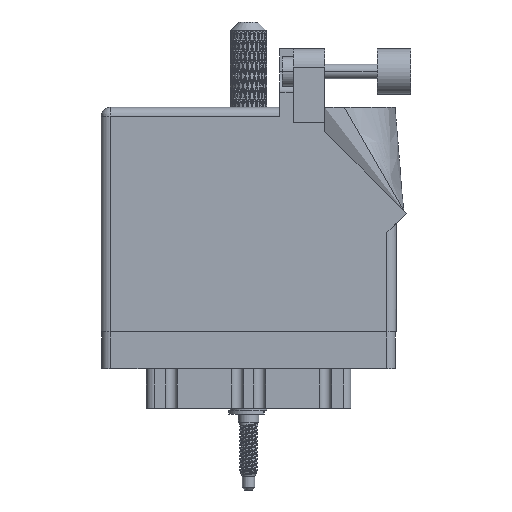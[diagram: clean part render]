
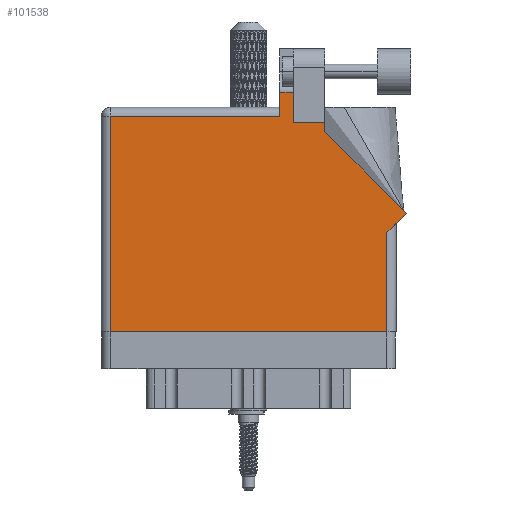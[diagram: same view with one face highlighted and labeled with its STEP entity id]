
A CAD part, front view. The second image highlights one B-rep face of the part: STEP entity #101538.
In plain terms, the highlighted face is planar.
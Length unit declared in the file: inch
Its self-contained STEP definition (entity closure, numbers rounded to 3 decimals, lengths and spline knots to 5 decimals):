
#59 = DIRECTION ( 'NONE',  ( -1., 0., 0. ) ) ;
#2060 = VERTEX_POINT ( 'NONE', #86287 ) ;
#2966 = CARTESIAN_POINT ( 'NONE',  ( 1.948, 0.675, 0. ) ) ;
#5149 = CARTESIAN_POINT ( 'NONE',  ( 2.08071, 0.80771, 0. ) ) ;
#6017 = EDGE_CURVE ( 'NONE', #79848, #96081, #8811, .T. ) ;
#7831 = ORIENTED_EDGE ( 'NONE', *, *, #81977, .T. ) ;
#8289 = CARTESIAN_POINT ( 'NONE',  ( 0., 1.468, 0. ) ) ;
#8692 = CARTESIAN_POINT ( 'NONE',  ( 0.062, 1.468, 0. ) ) ;
#8811 = LINE ( 'NONE', #8289, #60024 ) ;
#11763 = EDGE_CURVE ( 'NONE', #2060, #68552, #32461, .T. ) ;
#12787 = VECTOR ( 'NONE', #89440, 39.37008 ) ;
#12826 = VERTEX_POINT ( 'NONE', #76459 ) ;
#13745 = VECTOR ( 'NONE', #19058, 39.37008 ) ;
#13921 = LINE ( 'NONE', #80703, #87282 ) ;
#13922 = CARTESIAN_POINT ( 'NONE',  ( 0., 1.53, 0. ) ) ;
#14000 = ORIENTED_EDGE ( 'NONE', *, *, #46606, .T. ) ;
#14435 = PLANE ( 'NONE',  #76879 ) ;
#14499 = VECTOR ( 'NONE', #88847, 39.37008 ) ;
#15387 = ORIENTED_EDGE ( 'NONE', *, *, #80254, .T. ) ;
#15699 = LINE ( 'NONE', #31146, #12787 ) ;
#18017 = CARTESIAN_POINT ( 'NONE',  ( 1.524, 1.36442, 0. ) ) ;
#19058 = DIRECTION ( 'NONE',  ( 0., 1., 0. ) ) ;
#19302 = CARTESIAN_POINT ( 'NONE',  ( 1.311, 1.43, 0. ) ) ;
#19380 = LINE ( 'NONE', #28450, #73697 ) ;
#22245 = CARTESIAN_POINT ( 'NONE',  ( 2.08071, 0.80771, 0. ) ) ;
#24450 = EDGE_CURVE ( 'NONE', #85967, #58935, #13921, .T. ) ;
#26199 = ORIENTED_EDGE ( 'NONE', *, *, #64897, .T. ) ;
#26257 = LINE ( 'NONE', #19302, #26749 ) ;
#26749 = VECTOR ( 'NONE', #43212, 39.37008 ) ;
#28450 = CARTESIAN_POINT ( 'NONE',  ( 1.948, 0.737, 0. ) ) ;
#29911 = EDGE_CURVE ( 'NONE', #47731, #33781, #68970, .T. ) ;
#31067 = EDGE_CURVE ( 'NONE', #58935, #2060, #26257, .T. ) ;
#31146 = CARTESIAN_POINT ( 'NONE',  ( 0.062, 0., 0. ) ) ;
#31417 = FACE_OUTER_BOUND ( 'NONE', #61093, .T. ) ;
#32461 = LINE ( 'NONE', #50458, #50585 ) ;
#33781 = VERTEX_POINT ( 'NONE', #96773 ) ;
#35774 = ORIENTED_EDGE ( 'NONE', *, *, #31067, .T. ) ;
#37519 = DIRECTION ( 'NONE',  ( -0.707, 0.707, 0. ) ) ;
#40652 = DIRECTION ( 'NONE',  ( -1., 0., 0. ) ) ;
#43212 = DIRECTION ( 'NONE',  ( 0., 1., 0. ) ) ;
#43459 = ORIENTED_EDGE ( 'NONE', *, *, #24450, .T. ) ;
#45478 = LINE ( 'NONE', #5149, #87457 ) ;
#46606 = EDGE_CURVE ( 'NONE', #12826, #85967, #59933, .T. ) ;
#47731 = VERTEX_POINT ( 'NONE', #70955 ) ;
#50458 = CARTESIAN_POINT ( 'NONE',  ( 1.64177, 1.6315, 0. ) ) ;
#50585 = VECTOR ( 'NONE', #59, 39.37008 ) ;
#50645 = LINE ( 'NONE', #82974, #14499 ) ;
#52094 = VECTOR ( 'NONE', #56704, 39.37008 ) ;
#52248 = EDGE_CURVE ( 'NONE', #102484, #54928, #50645, .T. ) ;
#54928 = VERTEX_POINT ( 'NONE', #22245 ) ;
#56704 = DIRECTION ( 'NONE',  ( 0., -1., 0. ) ) ;
#58935 = VERTEX_POINT ( 'NONE', #88009 ) ;
#59933 = LINE ( 'NONE', #18017, #13745 ) ;
#60024 = VECTOR ( 'NONE', #40652, 39.37008 ) ;
#61093 = EDGE_LOOP ( 'NONE', ( #35774, #104684, #83140, #97493, #15387, #91819, #26199, #81775, #7831, #14000, #43459 ) ) ;
#61824 = DIRECTION ( 'NONE',  ( 0., 1., 0. ) ) ;
#64897 = EDGE_CURVE ( 'NONE', #33781, #102484, #19380, .T. ) ;
#65742 = LINE ( 'NONE', #97522, #52094 ) ;
#68552 = VERTEX_POINT ( 'NONE', #92241 ) ;
#68970 = LINE ( 'NONE', #86425, #104150 ) ;
#70955 = CARTESIAN_POINT ( 'NONE',  ( 0.062, 0., 0. ) ) ;
#73697 = VECTOR ( 'NONE', #61824, 39.37008 ) ;
#76459 = CARTESIAN_POINT ( 'NONE',  ( 1.524, 1.36442, 0. ) ) ;
#76879 = AXIS2_PLACEMENT_3D ( 'NONE', #13922, #94527, #96593 ) ;
#79848 = VERTEX_POINT ( 'NONE', #92431 ) ;
#80254 = EDGE_CURVE ( 'NONE', #96081, #47731, #15699, .T. ) ;
#80703 = CARTESIAN_POINT ( 'NONE',  ( 1.524, 1.43, 0. ) ) ;
#81775 = ORIENTED_EDGE ( 'NONE', *, *, #52248, .T. ) ;
#81977 = EDGE_CURVE ( 'NONE', #54928, #12826, #45478, .T. ) ;
#82974 = CARTESIAN_POINT ( 'NONE',  ( 2.01, 0.737, 0. ) ) ;
#83140 = ORIENTED_EDGE ( 'NONE', *, *, #89285, .T. ) ;
#85967 = VERTEX_POINT ( 'NONE', #93219 ) ;
#86287 = CARTESIAN_POINT ( 'NONE',  ( 1.311, 1.6315, 0. ) ) ;
#86425 = CARTESIAN_POINT ( 'NONE',  ( 0., 0., 0. ) ) ;
#87282 = VECTOR ( 'NONE', #95558, 39.37008 ) ;
#87457 = VECTOR ( 'NONE', #37519, 39.37008 ) ;
#88009 = CARTESIAN_POINT ( 'NONE',  ( 1.311, 1.43, 0. ) ) ;
#88847 = DIRECTION ( 'NONE',  ( 0.707, 0.707, 0. ) ) ;
#89285 = EDGE_CURVE ( 'NONE', #68552, #79848, #65742, .T. ) ;
#89440 = DIRECTION ( 'NONE',  ( 0., -1., 0. ) ) ;
#91819 = ORIENTED_EDGE ( 'NONE', *, *, #29911, .T. ) ;
#92241 = CARTESIAN_POINT ( 'NONE',  ( 1.217, 1.6315, 0. ) ) ;
#92431 = CARTESIAN_POINT ( 'NONE',  ( 1.217, 1.468, 0. ) ) ;
#93219 = CARTESIAN_POINT ( 'NONE',  ( 1.524, 1.43, 0. ) ) ;
#93829 = DIRECTION ( 'NONE',  ( 1., 0., 0. ) ) ;
#94527 = DIRECTION ( 'NONE',  ( 0., 0., -1. ) ) ;
#95558 = DIRECTION ( 'NONE',  ( -1., 0., 0. ) ) ;
#96081 = VERTEX_POINT ( 'NONE', #8692 ) ;
#96593 = DIRECTION ( 'NONE',  ( -1., 0., 0. ) ) ;
#96773 = CARTESIAN_POINT ( 'NONE',  ( 1.948, 0., 0. ) ) ;
#97493 = ORIENTED_EDGE ( 'NONE', *, *, #6017, .T. ) ;
#97522 = CARTESIAN_POINT ( 'NONE',  ( 1.217, 1.53, 0. ) ) ;
#101538 = ADVANCED_FACE ( 'NONE', ( #31417 ), #14435, .F. ) ;
#102484 = VERTEX_POINT ( 'NONE', #2966 ) ;
#104150 = VECTOR ( 'NONE', #93829, 39.37008 ) ;
#104684 = ORIENTED_EDGE ( 'NONE', *, *, #11763, .T. ) ;
